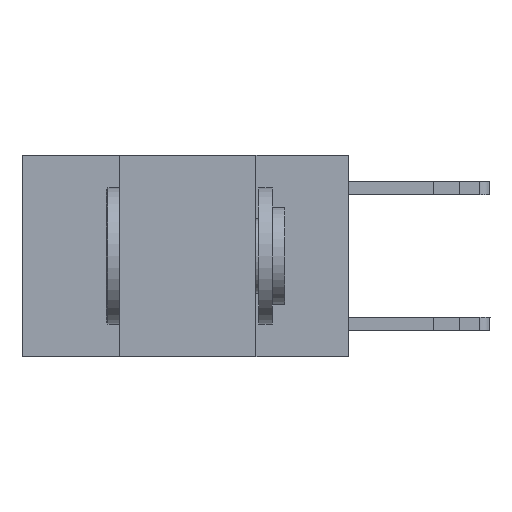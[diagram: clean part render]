
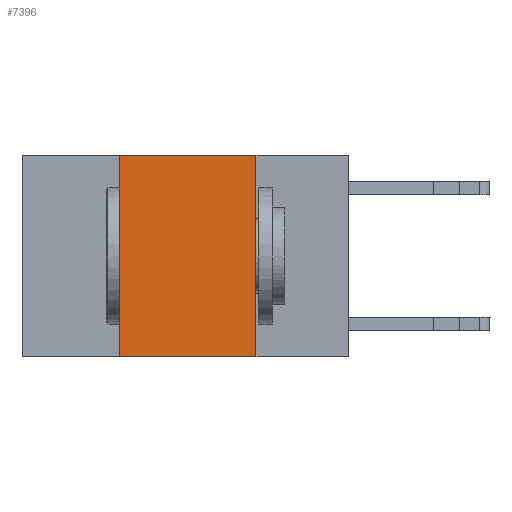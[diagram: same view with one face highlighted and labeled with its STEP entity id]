
A CAD part, left-side view. The second image highlights one B-rep face of the part: STEP entity #7396.
In plain terms, the highlighted planar face has unit normal (-1, 0, 0).
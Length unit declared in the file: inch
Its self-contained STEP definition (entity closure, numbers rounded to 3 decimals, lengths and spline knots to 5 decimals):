
#404 = DIRECTION ( 'NONE',  ( 0., -1., 0. ) ) ;
#832 = CARTESIAN_POINT ( 'NONE',  ( 0., 0.6, 0. ) ) ;
#864 = CARTESIAN_POINT ( 'NONE',  ( 0., 0.6, -0.37 ) ) ;
#1172 = PLANE ( 'NONE',  #6480 ) ;
#1225 = VECTOR ( 'NONE', #8131, 39.37008 ) ;
#1697 = VECTOR ( 'NONE', #17669, 39.37008 ) ;
#1717 = EDGE_CURVE ( 'NONE', #18873, #9644, #9513, .T. ) ;
#2061 = ORIENTED_EDGE ( 'NONE', *, *, #1717, .T. ) ;
#2390 = LINE ( 'NONE', #832, #1697 ) ;
#2765 = DIRECTION ( 'NONE',  ( 1., 0., 0. ) ) ;
#2919 = CARTESIAN_POINT ( 'NONE',  ( 0., 0.42, -0.37 ) ) ;
#4770 = LINE ( 'NONE', #5523, #5709 ) ;
#5450 = VERTEX_POINT ( 'NONE', #14545 ) ;
#5523 = CARTESIAN_POINT ( 'NONE',  ( 0., 0.42, 0. ) ) ;
#5709 = VECTOR ( 'NONE', #10105, 39.37008 ) ;
#6480 = AXIS2_PLACEMENT_3D ( 'NONE', #11893, #2765, #13449 ) ;
#6605 = CARTESIAN_POINT ( 'NONE',  ( 0., 0.17, 0. ) ) ;
#7396 = ADVANCED_FACE ( 'NONE', ( #12889 ), #1172, .F. ) ;
#8131 = DIRECTION ( 'NONE',  ( 0., 0., -1. ) ) ;
#9513 = LINE ( 'NONE', #864, #9992 ) ;
#9632 = EDGE_CURVE ( 'NONE', #16249, #5450, #2390, .T. ) ;
#9644 = VERTEX_POINT ( 'NONE', #10032 ) ;
#9992 = VECTOR ( 'NONE', #404, 39.37008 ) ;
#10032 = CARTESIAN_POINT ( 'NONE',  ( 0., 0.17, -0.37 ) ) ;
#10105 = DIRECTION ( 'NONE',  ( 0., 0., 1. ) ) ;
#11571 = EDGE_CURVE ( 'NONE', #18873, #16249, #4770, .T. ) ;
#11893 = CARTESIAN_POINT ( 'NONE',  ( 0., 0.6, 0. ) ) ;
#12288 = EDGE_LOOP ( 'NONE', ( #19403, #19601, #16276, #2061 ) ) ;
#12889 = FACE_OUTER_BOUND ( 'NONE', #12288, .T. ) ;
#13449 = DIRECTION ( 'NONE',  ( 0., 0., -1. ) ) ;
#13468 = LINE ( 'NONE', #6605, #1225 ) ;
#14545 = CARTESIAN_POINT ( 'NONE',  ( 0., 0.17, 0. ) ) ;
#16249 = VERTEX_POINT ( 'NONE', #16609 ) ;
#16276 = ORIENTED_EDGE ( 'NONE', *, *, #11571, .F. ) ;
#16609 = CARTESIAN_POINT ( 'NONE',  ( 0., 0.42, 0. ) ) ;
#17669 = DIRECTION ( 'NONE',  ( 0., -1., 0. ) ) ;
#18873 = VERTEX_POINT ( 'NONE', #2919 ) ;
#19114 = EDGE_CURVE ( 'NONE', #5450, #9644, #13468, .T. ) ;
#19403 = ORIENTED_EDGE ( 'NONE', *, *, #19114, .F. ) ;
#19601 = ORIENTED_EDGE ( 'NONE', *, *, #9632, .F. ) ;
